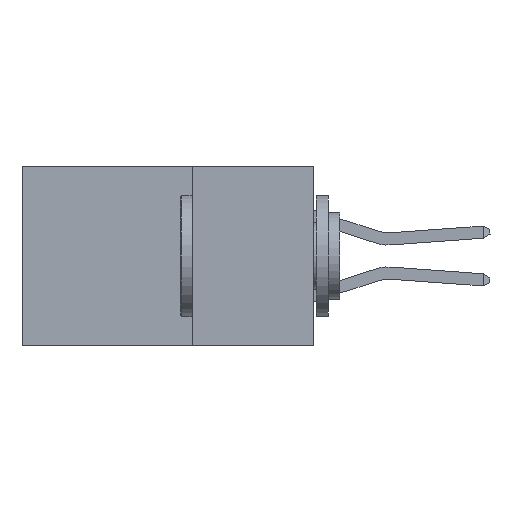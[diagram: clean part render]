
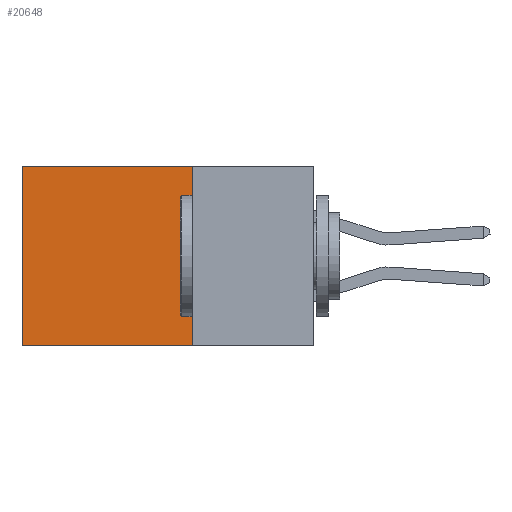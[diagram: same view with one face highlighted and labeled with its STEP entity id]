
A CAD part, left-side view. The second image highlights one B-rep face of the part: STEP entity #20648.
In plain terms, the highlighted planar face has unit normal (-1, 0, 0).
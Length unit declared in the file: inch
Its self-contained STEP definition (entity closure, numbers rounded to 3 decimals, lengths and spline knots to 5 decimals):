
#1844 = EDGE_LOOP ( 'NONE', ( #25527, #4807, #15917, #27058 ) ) ;
#2717 = EDGE_CURVE ( 'NONE', #15282, #29453, #33472, .T. ) ;
#3103 = CARTESIAN_POINT ( 'NONE',  ( 0.2875, 0.6, 0. ) ) ;
#4220 = DIRECTION ( 'NONE',  ( 0., 0., -1. ) ) ;
#4807 = ORIENTED_EDGE ( 'NONE', *, *, #20725, .F. ) ;
#5748 = CARTESIAN_POINT ( 'NONE',  ( 0.2875, 0.6, 0. ) ) ;
#5896 = LINE ( 'NONE', #14751, #28358 ) ;
#7191 = CARTESIAN_POINT ( 'NONE',  ( 0.2875, 0.25, -0.37 ) ) ;
#8070 = EDGE_CURVE ( 'NONE', #15282, #18381, #34517, .T. ) ;
#8467 = PLANE ( 'NONE',  #16680 ) ;
#8491 = CARTESIAN_POINT ( 'NONE',  ( 0.2875, 0.6, -0.37 ) ) ;
#8659 = DIRECTION ( 'NONE',  ( 0., 1., 0. ) ) ;
#9527 = CARTESIAN_POINT ( 'NONE',  ( 0.2875, 0.25, 0. ) ) ;
#12309 = VECTOR ( 'NONE', #30341, 39.37008 ) ;
#12924 = VECTOR ( 'NONE', #8659, 39.37008 ) ;
#14540 = VERTEX_POINT ( 'NONE', #8491 ) ;
#14751 = CARTESIAN_POINT ( 'NONE',  ( 0.2875, 0.25, -0.37 ) ) ;
#15282 = VERTEX_POINT ( 'NONE', #34836 ) ;
#15917 = ORIENTED_EDGE ( 'NONE', *, *, #2717, .F. ) ;
#16680 = AXIS2_PLACEMENT_3D ( 'NONE', #27557, #19275, #19621 ) ;
#16727 = CARTESIAN_POINT ( 'NONE',  ( 0.2875, 0.25, 0. ) ) ;
#18381 = VERTEX_POINT ( 'NONE', #5748 ) ;
#19275 = DIRECTION ( 'NONE',  ( 1., 0., 0. ) ) ;
#19621 = DIRECTION ( 'NONE',  ( 0., 0., -1. ) ) ;
#20648 = ADVANCED_FACE ( 'NONE', ( #33419 ), #8467, .F. ) ;
#20725 = EDGE_CURVE ( 'NONE', #29453, #14540, #5896, .T. ) ;
#25527 = ORIENTED_EDGE ( 'NONE', *, *, #34183, .T. ) ;
#27058 = ORIENTED_EDGE ( 'NONE', *, *, #8070, .T. ) ;
#27552 = VECTOR ( 'NONE', #4220, 39.37008 ) ;
#27557 = CARTESIAN_POINT ( 'NONE',  ( 0.2875, 0.25, 0. ) ) ;
#28358 = VECTOR ( 'NONE', #33803, 39.37008 ) ;
#29453 = VERTEX_POINT ( 'NONE', #7191 ) ;
#30341 = DIRECTION ( 'NONE',  ( 0., 0., -1. ) ) ;
#33419 = FACE_OUTER_BOUND ( 'NONE', #1844, .T. ) ;
#33472 = LINE ( 'NONE', #9527, #27552 ) ;
#33803 = DIRECTION ( 'NONE',  ( 0., 1., 0. ) ) ;
#34183 = EDGE_CURVE ( 'NONE', #18381, #14540, #34286, .T. ) ;
#34286 = LINE ( 'NONE', #3103, #12309 ) ;
#34517 = LINE ( 'NONE', #16727, #12924 ) ;
#34836 = CARTESIAN_POINT ( 'NONE',  ( 0.2875, 0.25, 0. ) ) ;
